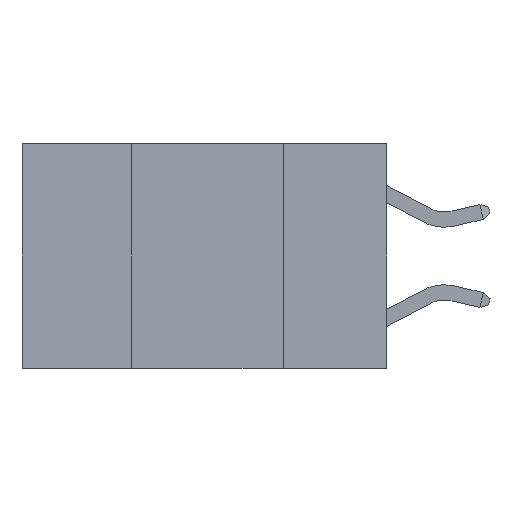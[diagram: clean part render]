
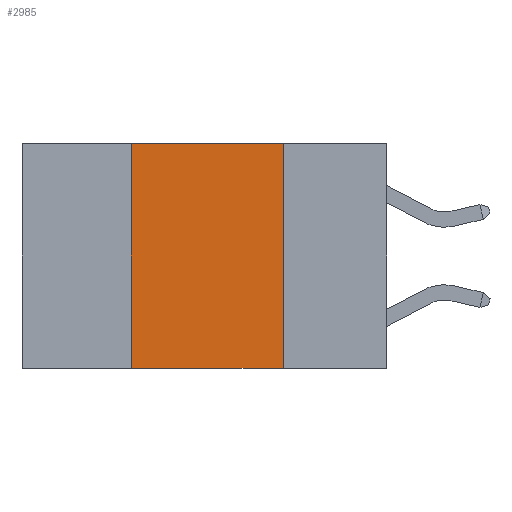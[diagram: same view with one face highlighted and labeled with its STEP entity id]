
A CAD part, left-side view. The second image highlights one B-rep face of the part: STEP entity #2985.
In plain terms, the highlighted planar face has unit normal (-1, 0, 0).
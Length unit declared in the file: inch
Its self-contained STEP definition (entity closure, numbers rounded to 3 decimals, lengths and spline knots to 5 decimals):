
#796 = ORIENTED_EDGE ( 'NONE', *, *, #5131, .T. ) ;
#1154 = VERTEX_POINT ( 'NONE', #8050 ) ;
#1423 = VECTOR ( 'NONE', #16651, 39.37008 ) ;
#2985 = ADVANCED_FACE ( 'NONE', ( #9055 ), #25379, .F. ) ;
#3736 = CARTESIAN_POINT ( 'NONE',  ( 0., 0.42, 0. ) ) ;
#3858 = LINE ( 'NONE', #3736, #1423 ) ;
#5117 = ORIENTED_EDGE ( 'NONE', *, *, #6179, .F. ) ;
#5131 = EDGE_CURVE ( 'NONE', #1154, #25313, #5713, .T. ) ;
#5425 = CARTESIAN_POINT ( 'NONE',  ( 0., 0.17, 0. ) ) ;
#5713 = LINE ( 'NONE', #18618, #7378 ) ;
#6179 = EDGE_CURVE ( 'NONE', #1154, #22509, #3858, .T. ) ;
#6284 = ORIENTED_EDGE ( 'NONE', *, *, #11186, .F. ) ;
#7145 = DIRECTION ( 'NONE',  ( 0., -1., 0. ) ) ;
#7378 = VECTOR ( 'NONE', #27011, 39.37008 ) ;
#8050 = CARTESIAN_POINT ( 'NONE',  ( 0., 0.42, -0.37 ) ) ;
#8791 = CARTESIAN_POINT ( 'NONE',  ( 0., 0.17, -0.37 ) ) ;
#9055 = FACE_OUTER_BOUND ( 'NONE', #20903, .T. ) ;
#9086 = CARTESIAN_POINT ( 'NONE',  ( 0., 0.6, 0. ) ) ;
#10642 = EDGE_CURVE ( 'NONE', #22509, #20707, #11155, .T. ) ;
#11155 = LINE ( 'NONE', #9086, #11202 ) ;
#11186 = EDGE_CURVE ( 'NONE', #20707, #25313, #13975, .T. ) ;
#11202 = VECTOR ( 'NONE', #7145, 39.37008 ) ;
#13404 = VECTOR ( 'NONE', #22359, 39.37008 ) ;
#13975 = LINE ( 'NONE', #24555, #13404 ) ;
#14960 = DIRECTION ( 'NONE',  ( 0., 0., -1. ) ) ;
#16651 = DIRECTION ( 'NONE',  ( 0., 0., 1. ) ) ;
#16991 = AXIS2_PLACEMENT_3D ( 'NONE', #23340, #21677, #14960 ) ;
#17744 = ORIENTED_EDGE ( 'NONE', *, *, #10642, .F. ) ;
#18618 = CARTESIAN_POINT ( 'NONE',  ( 0., 0.6, -0.37 ) ) ;
#20707 = VERTEX_POINT ( 'NONE', #5425 ) ;
#20903 = EDGE_LOOP ( 'NONE', ( #6284, #17744, #5117, #796 ) ) ;
#21677 = DIRECTION ( 'NONE',  ( 1., 0., 0. ) ) ;
#22359 = DIRECTION ( 'NONE',  ( 0., 0., -1. ) ) ;
#22509 = VERTEX_POINT ( 'NONE', #24750 ) ;
#23340 = CARTESIAN_POINT ( 'NONE',  ( 0., 0.6, 0. ) ) ;
#24555 = CARTESIAN_POINT ( 'NONE',  ( 0., 0.17, 0. ) ) ;
#24750 = CARTESIAN_POINT ( 'NONE',  ( 0., 0.42, 0. ) ) ;
#25313 = VERTEX_POINT ( 'NONE', #8791 ) ;
#25379 = PLANE ( 'NONE',  #16991 ) ;
#27011 = DIRECTION ( 'NONE',  ( 0., -1., 0. ) ) ;
